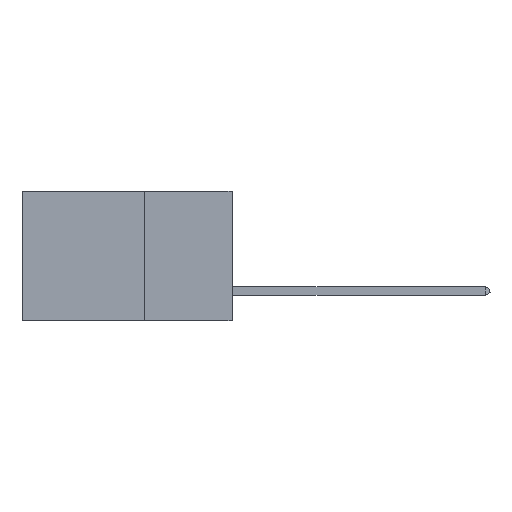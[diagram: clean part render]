
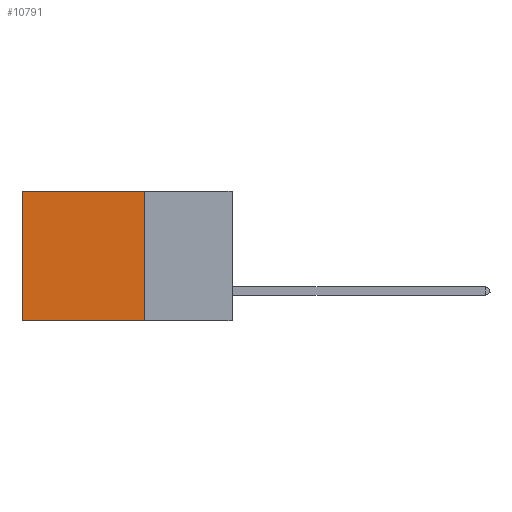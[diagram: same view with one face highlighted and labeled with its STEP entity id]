
A CAD part, left-side view. The second image highlights one B-rep face of the part: STEP entity #10791.
In plain terms, the highlighted planar face has unit normal (-1, 0, 0).
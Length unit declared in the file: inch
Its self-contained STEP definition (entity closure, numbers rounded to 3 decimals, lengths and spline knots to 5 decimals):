
#263 = CARTESIAN_POINT ( 'NONE',  ( 0.2875, 0.6, 0. ) ) ;
#503 = ORIENTED_EDGE ( 'NONE', *, *, #4733, .T. ) ;
#564 = EDGE_LOOP ( 'NONE', ( #503, #6133, #8459, #11336 ) ) ;
#1456 = VECTOR ( 'NONE', #13014, 39.37008 ) ;
#1502 = DIRECTION ( 'NONE',  ( 0., 1., 0. ) ) ;
#2057 = EDGE_CURVE ( 'NONE', #3838, #6987, #10264, .T. ) ;
#2439 = VERTEX_POINT ( 'NONE', #9752 ) ;
#3163 = CARTESIAN_POINT ( 'NONE',  ( 0.2875, 0.25, 0. ) ) ;
#3838 = VERTEX_POINT ( 'NONE', #10471 ) ;
#4733 = EDGE_CURVE ( 'NONE', #8779, #6987, #10381, .T. ) ;
#4784 = EDGE_CURVE ( 'NONE', #2439, #8779, #9985, .T. ) ;
#6133 = ORIENTED_EDGE ( 'NONE', *, *, #2057, .F. ) ;
#6833 = VECTOR ( 'NONE', #13307, 39.37008 ) ;
#6987 = VERTEX_POINT ( 'NONE', #12561 ) ;
#7952 = VECTOR ( 'NONE', #1502, 39.37008 ) ;
#8208 = PLANE ( 'NONE',  #10546 ) ;
#8459 = ORIENTED_EDGE ( 'NONE', *, *, #9320, .F. ) ;
#8758 = CARTESIAN_POINT ( 'NONE',  ( 0.2875, 0.25, -0.37 ) ) ;
#8779 = VERTEX_POINT ( 'NONE', #14647 ) ;
#9277 = FACE_OUTER_BOUND ( 'NONE', #564, .T. ) ;
#9320 = EDGE_CURVE ( 'NONE', #2439, #3838, #16406, .T. ) ;
#9752 = CARTESIAN_POINT ( 'NONE',  ( 0.2875, 0.25, 0. ) ) ;
#9918 = VECTOR ( 'NONE', #10216, 39.37008 ) ;
#9985 = LINE ( 'NONE', #14525, #7952 ) ;
#10216 = DIRECTION ( 'NONE',  ( 0., 0., -1. ) ) ;
#10264 = LINE ( 'NONE', #8758, #6833 ) ;
#10381 = LINE ( 'NONE', #263, #1456 ) ;
#10471 = CARTESIAN_POINT ( 'NONE',  ( 0.2875, 0.25, -0.37 ) ) ;
#10546 = AXIS2_PLACEMENT_3D ( 'NONE', #3163, #12068, #14806 ) ;
#10791 = ADVANCED_FACE ( 'NONE', ( #9277 ), #8208, .F. ) ;
#11336 = ORIENTED_EDGE ( 'NONE', *, *, #4784, .T. ) ;
#12068 = DIRECTION ( 'NONE',  ( 1., 0., 0. ) ) ;
#12561 = CARTESIAN_POINT ( 'NONE',  ( 0.2875, 0.6, -0.37 ) ) ;
#12772 = CARTESIAN_POINT ( 'NONE',  ( 0.2875, 0.25, 0. ) ) ;
#13014 = DIRECTION ( 'NONE',  ( 0., 0., -1. ) ) ;
#13307 = DIRECTION ( 'NONE',  ( 0., 1., 0. ) ) ;
#14525 = CARTESIAN_POINT ( 'NONE',  ( 0.2875, 0.25, 0. ) ) ;
#14647 = CARTESIAN_POINT ( 'NONE',  ( 0.2875, 0.6, 0. ) ) ;
#14806 = DIRECTION ( 'NONE',  ( 0., 0., -1. ) ) ;
#16406 = LINE ( 'NONE', #12772, #9918 ) ;
